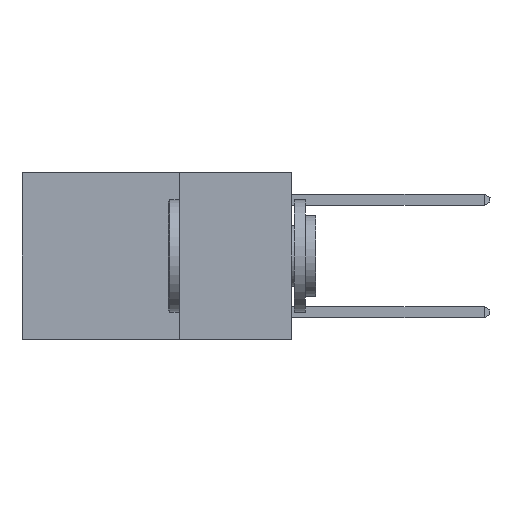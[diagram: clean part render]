
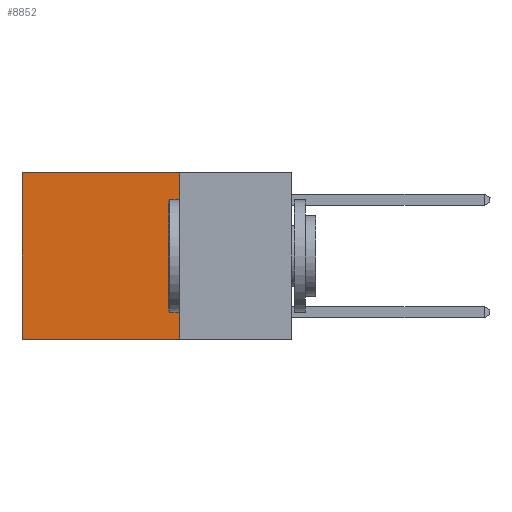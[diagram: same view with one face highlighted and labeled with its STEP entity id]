
A CAD part, left-side view. The second image highlights one B-rep face of the part: STEP entity #8852.
In plain terms, the highlighted planar face has unit normal (-1, 0, 0).
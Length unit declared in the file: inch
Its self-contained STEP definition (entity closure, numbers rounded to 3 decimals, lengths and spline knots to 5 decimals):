
#1032 = CARTESIAN_POINT ( 'NONE',  ( 0.2625, 0.6, 0. ) ) ;
#1810 = DIRECTION ( 'NONE',  ( 0., 0., -1. ) ) ;
#1877 = FACE_OUTER_BOUND ( 'NONE', #4114, .T. ) ;
#1896 = EDGE_CURVE ( 'NONE', #7583, #4030, #5093, .T. ) ;
#2103 = DIRECTION ( 'NONE',  ( 0., 0., -1. ) ) ;
#2868 = VECTOR ( 'NONE', #10554, 39.37008 ) ;
#2955 = LINE ( 'NONE', #5331, #13148 ) ;
#3902 = EDGE_CURVE ( 'NONE', #5091, #10611, #8418, .T. ) ;
#4030 = VERTEX_POINT ( 'NONE', #1032 ) ;
#4114 = EDGE_LOOP ( 'NONE', ( #9967, #7698, #9530, #12124 ) ) ;
#4529 = LINE ( 'NONE', #10015, #10079 ) ;
#5091 = VERTEX_POINT ( 'NONE', #11025 ) ;
#5093 = LINE ( 'NONE', #6227, #2868 ) ;
#5156 = DIRECTION ( 'NONE',  ( 1., 0., 0. ) ) ;
#5331 = CARTESIAN_POINT ( 'NONE',  ( 0.2625, 0.25, 0. ) ) ;
#5458 = EDGE_CURVE ( 'NONE', #7583, #5091, #2955, .T. ) ;
#6227 = CARTESIAN_POINT ( 'NONE',  ( 0.2625, 0.25, 0. ) ) ;
#7583 = VERTEX_POINT ( 'NONE', #13118 ) ;
#7698 = ORIENTED_EDGE ( 'NONE', *, *, #3902, .F. ) ;
#8103 = VECTOR ( 'NONE', #8280, 39.37008 ) ;
#8280 = DIRECTION ( 'NONE',  ( 0., 1., 0. ) ) ;
#8418 = LINE ( 'NONE', #10424, #8103 ) ;
#8462 = CARTESIAN_POINT ( 'NONE',  ( 0.2625, 0.6, -0.37 ) ) ;
#8722 = DIRECTION ( 'NONE',  ( 0., 0., -1. ) ) ;
#8852 = ADVANCED_FACE ( 'NONE', ( #1877 ), #11753, .F. ) ;
#9530 = ORIENTED_EDGE ( 'NONE', *, *, #5458, .F. ) ;
#9967 = ORIENTED_EDGE ( 'NONE', *, *, #13482, .T. ) ;
#10015 = CARTESIAN_POINT ( 'NONE',  ( 0.2625, 0.6, 0. ) ) ;
#10079 = VECTOR ( 'NONE', #8722, 39.37008 ) ;
#10424 = CARTESIAN_POINT ( 'NONE',  ( 0.2625, 0.25, -0.37 ) ) ;
#10554 = DIRECTION ( 'NONE',  ( 0., 1., 0. ) ) ;
#10611 = VERTEX_POINT ( 'NONE', #8462 ) ;
#11025 = CARTESIAN_POINT ( 'NONE',  ( 0.2625, 0.25, -0.37 ) ) ;
#11556 = CARTESIAN_POINT ( 'NONE',  ( 0.2625, 0.25, 0. ) ) ;
#11753 = PLANE ( 'NONE',  #13633 ) ;
#12124 = ORIENTED_EDGE ( 'NONE', *, *, #1896, .T. ) ;
#13118 = CARTESIAN_POINT ( 'NONE',  ( 0.2625, 0.25, 0. ) ) ;
#13148 = VECTOR ( 'NONE', #2103, 39.37008 ) ;
#13482 = EDGE_CURVE ( 'NONE', #4030, #10611, #4529, .T. ) ;
#13633 = AXIS2_PLACEMENT_3D ( 'NONE', #11556, #5156, #1810 ) ;
